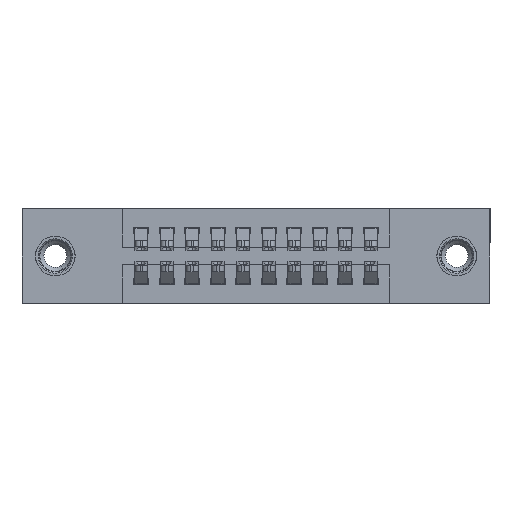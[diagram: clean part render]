
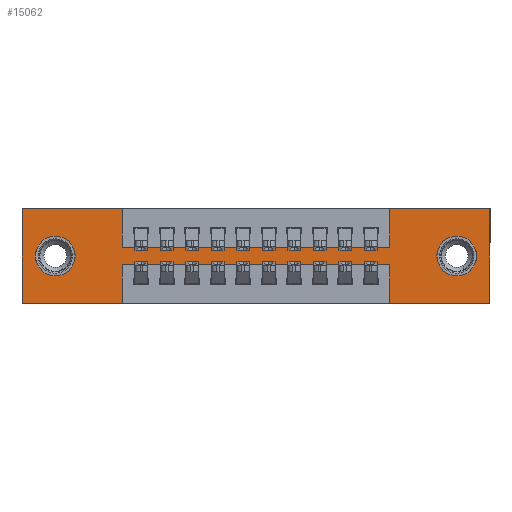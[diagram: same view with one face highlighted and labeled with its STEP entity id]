
A CAD part, front view. The second image highlights one B-rep face of the part: STEP entity #15062.
In plain terms, the highlighted planar face has unit normal (0, -1, 0).
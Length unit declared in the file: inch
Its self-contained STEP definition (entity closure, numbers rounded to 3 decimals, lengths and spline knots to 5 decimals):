
#243 = CARTESIAN_POINT ( 'NONE',  ( 0., 0., -0.37 ) ) ;
#257 = ORIENTED_EDGE ( 'NONE', *, *, #2554, .F. ) ;
#276 = ORIENTED_EDGE ( 'NONE', *, *, #4396, .F. ) ;
#324 = EDGE_LOOP ( 'NONE', ( #9780, #2620 ) ) ;
#594 = ORIENTED_EDGE ( 'NONE', *, *, #1978, .T. ) ;
#602 = LINE ( 'NONE', #3804, #6546 ) ;
#850 = FACE_OUTER_BOUND ( 'NONE', #3905, .T. ) ;
#868 = DIRECTION ( 'NONE',  ( 0., 0., -1. ) ) ;
#1363 = VERTEX_POINT ( 'NONE', #13252 ) ;
#1563 = ORIENTED_EDGE ( 'NONE', *, *, #10762, .T. ) ;
#1619 = VERTEX_POINT ( 'NONE', #2670 ) ;
#1635 = LINE ( 'NONE', #7882, #5701 ) ;
#1978 = EDGE_CURVE ( 'NONE', #2266, #1363, #8524, .T. ) ;
#2017 = LINE ( 'NONE', #12880, #12303 ) ;
#2227 = ORIENTED_EDGE ( 'NONE', *, *, #12169, .F. ) ;
#2266 = VERTEX_POINT ( 'NONE', #5858 ) ;
#2292 = CARTESIAN_POINT ( 'NONE',  ( 0.13, 0., -0.185 ) ) ;
#2314 = ORIENTED_EDGE ( 'NONE', *, *, #14480, .F. ) ;
#2331 = DIRECTION ( 'NONE',  ( 0., -1., 0. ) ) ;
#2334 = ORIENTED_EDGE ( 'NONE', *, *, #8775, .F. ) ;
#2413 = ORIENTED_EDGE ( 'NONE', *, *, #9671, .F. ) ;
#2554 = EDGE_CURVE ( 'NONE', #14967, #6202, #14658, .T. ) ;
#2620 = ORIENTED_EDGE ( 'NONE', *, *, #14324, .T. ) ;
#2665 = CARTESIAN_POINT ( 'NONE',  ( 0., 0., -0.37 ) ) ;
#2670 = CARTESIAN_POINT ( 'NONE',  ( 0.3925, 0., 0. ) ) ;
#2757 = AXIS2_PLACEMENT_3D ( 'NONE', #3664, #2331, #11707 ) ;
#2993 = ORIENTED_EDGE ( 'NONE', *, *, #8723, .F. ) ;
#3036 = LINE ( 'NONE', #13276, #5786 ) ;
#3038 = VERTEX_POINT ( 'NONE', #12413 ) ;
#3048 = CARTESIAN_POINT ( 'NONE',  ( 1.835, 0., -0.37 ) ) ;
#3061 = ORIENTED_EDGE ( 'NONE', *, *, #12995, .F. ) ;
#3322 = ORIENTED_EDGE ( 'NONE', *, *, #7286, .F. ) ;
#3502 = VECTOR ( 'NONE', #8804, 39.37008 ) ;
#3636 = AXIS2_PLACEMENT_3D ( 'NONE', #4049, #13335, #5400 ) ;
#3664 = CARTESIAN_POINT ( 'NONE',  ( 0., 0., -0.37 ) ) ;
#3687 = DIRECTION ( 'NONE',  ( 0., 0., 1. ) ) ;
#3735 = CIRCLE ( 'NONE', #12747, 0.078 ) ;
#3745 = DIRECTION ( 'NONE',  ( 0., 0., -1. ) ) ;
#3755 = AXIS2_PLACEMENT_3D ( 'NONE', #2292, #11669, #3687 ) ;
#3804 = CARTESIAN_POINT ( 'NONE',  ( 1.835, 0., 0. ) ) ;
#3808 = EDGE_CURVE ( 'NONE', #1619, #15254, #14004, .T. ) ;
#3858 = EDGE_CURVE ( 'NONE', #5129, #4149, #602, .T. ) ;
#3905 = EDGE_LOOP ( 'NONE', ( #2993, #3061, #3322, #2227, #4320, #5191, #2314, #2334, #4536, #2413, #257, #276 ) ) ;
#3941 = EDGE_LOOP ( 'NONE', ( #594, #1563 ) ) ;
#4049 = CARTESIAN_POINT ( 'NONE',  ( 0.13, 0., -0.185 ) ) ;
#4149 = VERTEX_POINT ( 'NONE', #3048 ) ;
#4315 = DIRECTION ( 'NONE',  ( -1., 0., 0. ) ) ;
#4320 = ORIENTED_EDGE ( 'NONE', *, *, #3858, .F. ) ;
#4396 = EDGE_CURVE ( 'NONE', #3038, #14967, #16436, .T. ) ;
#4428 = AXIS2_PLACEMENT_3D ( 'NONE', #5921, #6416, #868 ) ;
#4519 = CARTESIAN_POINT ( 'NONE',  ( 0.13, 0., -0.107 ) ) ;
#4536 = ORIENTED_EDGE ( 'NONE', *, *, #3808, .F. ) ;
#4612 = VERTEX_POINT ( 'NONE', #5814 ) ;
#4999 = VERTEX_POINT ( 'NONE', #14579 ) ;
#5129 = VERTEX_POINT ( 'NONE', #9556 ) ;
#5172 = DIRECTION ( 'NONE',  ( 0., 0., -1. ) ) ;
#5191 = ORIENTED_EDGE ( 'NONE', *, *, #14303, .F. ) ;
#5400 = DIRECTION ( 'NONE',  ( 0., 0., 1. ) ) ;
#5701 = VECTOR ( 'NONE', #17027, 39.37008 ) ;
#5786 = VECTOR ( 'NONE', #14714, 39.37008 ) ;
#5814 = CARTESIAN_POINT ( 'NONE',  ( 1.4425, 0., -0.15 ) ) ;
#5858 = CARTESIAN_POINT ( 'NONE',  ( 1.705, 0., -0.107 ) ) ;
#5921 = CARTESIAN_POINT ( 'NONE',  ( 1.705, 0., -0.185 ) ) ;
#6202 = VERTEX_POINT ( 'NONE', #9156 ) ;
#6337 = CARTESIAN_POINT ( 'NONE',  ( 0., 0., 0. ) ) ;
#6394 = DIRECTION ( 'NONE',  ( 0., 0., -1. ) ) ;
#6402 = CIRCLE ( 'NONE', #3636, 0.078 ) ;
#6416 = DIRECTION ( 'NONE',  ( 0., 1., 0. ) ) ;
#6546 = VECTOR ( 'NONE', #5172, 39.37008 ) ;
#6795 = CARTESIAN_POINT ( 'NONE',  ( 0.3925, 0., -0.15 ) ) ;
#7286 = EDGE_CURVE ( 'NONE', #10394, #16884, #15423, .T. ) ;
#7511 = CARTESIAN_POINT ( 'NONE',  ( 1.705, 0., -0.185 ) ) ;
#7737 = PLANE ( 'NONE',  #2757 ) ;
#7882 = CARTESIAN_POINT ( 'NONE',  ( 0.3925, 0., -0.15 ) ) ;
#7884 = LINE ( 'NONE', #6337, #14871 ) ;
#8087 = FACE_BOUND ( 'NONE', #324, .T. ) ;
#8226 = CARTESIAN_POINT ( 'NONE',  ( 1.4425, 0., -0.22 ) ) ;
#8509 = VECTOR ( 'NONE', #16335, 39.37008 ) ;
#8524 = CIRCLE ( 'NONE', #4428, 0.078 ) ;
#8605 = VERTEX_POINT ( 'NONE', #8769 ) ;
#8723 = EDGE_CURVE ( 'NONE', #11041, #3038, #9687, .T. ) ;
#8769 = CARTESIAN_POINT ( 'NONE',  ( 0.13, 0., -0.263 ) ) ;
#8775 = EDGE_CURVE ( 'NONE', #15254, #4612, #1635, .T. ) ;
#8804 = DIRECTION ( 'NONE',  ( -1., 0., 0. ) ) ;
#8850 = DIRECTION ( 'NONE',  ( 0., 0., -1. ) ) ;
#9045 = CARTESIAN_POINT ( 'NONE',  ( 1.4425, 0., -0.37 ) ) ;
#9156 = CARTESIAN_POINT ( 'NONE',  ( 0., 0., 0. ) ) ;
#9466 = DIRECTION ( 'NONE',  ( 0., 0., 1. ) ) ;
#9556 = CARTESIAN_POINT ( 'NONE',  ( 1.835, 0., 0. ) ) ;
#9671 = EDGE_CURVE ( 'NONE', #6202, #1619, #2017, .T. ) ;
#9687 = LINE ( 'NONE', #15601, #13136 ) ;
#9780 = ORIENTED_EDGE ( 'NONE', *, *, #12649, .T. ) ;
#9996 = LINE ( 'NONE', #243, #13881 ) ;
#10325 = VECTOR ( 'NONE', #12008, 39.37008 ) ;
#10394 = VERTEX_POINT ( 'NONE', #9045 ) ;
#10762 = EDGE_CURVE ( 'NONE', #1363, #2266, #3735, .T. ) ;
#11041 = VERTEX_POINT ( 'NONE', #13304 ) ;
#11388 = CIRCLE ( 'NONE', #3755, 0.078 ) ;
#11669 = DIRECTION ( 'NONE',  ( 0., 1., 0. ) ) ;
#11707 = DIRECTION ( 'NONE',  ( 0., 0., -1. ) ) ;
#11735 = CARTESIAN_POINT ( 'NONE',  ( 0.3925, 0., 0. ) ) ;
#11957 = VECTOR ( 'NONE', #9466, 39.37008 ) ;
#12008 = DIRECTION ( 'NONE',  ( -1., 0., 0. ) ) ;
#12169 = EDGE_CURVE ( 'NONE', #4149, #10394, #9996, .T. ) ;
#12303 = VECTOR ( 'NONE', #12937, 39.37008 ) ;
#12413 = CARTESIAN_POINT ( 'NONE',  ( 0.3925, 0., -0.37 ) ) ;
#12649 = EDGE_CURVE ( 'NONE', #12871, #8605, #6402, .T. ) ;
#12747 = AXIS2_PLACEMENT_3D ( 'NONE', #7511, #16661, #8850 ) ;
#12795 = CARTESIAN_POINT ( 'NONE',  ( 0., 0., -0.37 ) ) ;
#12871 = VERTEX_POINT ( 'NONE', #4519 ) ;
#12880 = CARTESIAN_POINT ( 'NONE',  ( 0., 0., 0. ) ) ;
#12937 = DIRECTION ( 'NONE',  ( 1., 0., 0. ) ) ;
#12995 = EDGE_CURVE ( 'NONE', #16884, #11041, #13699, .T. ) ;
#13136 = VECTOR ( 'NONE', #6394, 39.37008 ) ;
#13252 = CARTESIAN_POINT ( 'NONE',  ( 1.705, 0., -0.263 ) ) ;
#13276 = CARTESIAN_POINT ( 'NONE',  ( 1.4425, 0., 0. ) ) ;
#13304 = CARTESIAN_POINT ( 'NONE',  ( 0.3925, 0., -0.22 ) ) ;
#13335 = DIRECTION ( 'NONE',  ( 0., 1., 0. ) ) ;
#13699 = LINE ( 'NONE', #15363, #3502 ) ;
#13881 = VECTOR ( 'NONE', #4315, 39.37008 ) ;
#14004 = LINE ( 'NONE', #11735, #14417 ) ;
#14303 = EDGE_CURVE ( 'NONE', #4999, #5129, #7884, .T. ) ;
#14324 = EDGE_CURVE ( 'NONE', #8605, #12871, #11388, .T. ) ;
#14417 = VECTOR ( 'NONE', #3745, 39.37008 ) ;
#14480 = EDGE_CURVE ( 'NONE', #4612, #4999, #3036, .T. ) ;
#14579 = CARTESIAN_POINT ( 'NONE',  ( 1.4425, 0., 0. ) ) ;
#14650 = FACE_BOUND ( 'NONE', #3941, .T. ) ;
#14658 = LINE ( 'NONE', #16521, #8509 ) ;
#14661 = CARTESIAN_POINT ( 'NONE',  ( 1.4425, 0., -0.37 ) ) ;
#14714 = DIRECTION ( 'NONE',  ( 0., 0., 1. ) ) ;
#14871 = VECTOR ( 'NONE', #15542, 39.37008 ) ;
#14967 = VERTEX_POINT ( 'NONE', #12795 ) ;
#15062 = ADVANCED_FACE ( 'NONE', ( #14650, #8087, #850 ), #7737, .T. ) ;
#15254 = VERTEX_POINT ( 'NONE', #6795 ) ;
#15363 = CARTESIAN_POINT ( 'NONE',  ( 0.3925, 0., -0.22 ) ) ;
#15423 = LINE ( 'NONE', #14661, #11957 ) ;
#15542 = DIRECTION ( 'NONE',  ( 1., 0., 0. ) ) ;
#15601 = CARTESIAN_POINT ( 'NONE',  ( 0.3925, 0., -0.37 ) ) ;
#16335 = DIRECTION ( 'NONE',  ( 0., 0., 1. ) ) ;
#16436 = LINE ( 'NONE', #2665, #10325 ) ;
#16521 = CARTESIAN_POINT ( 'NONE',  ( 0., 0., 0. ) ) ;
#16661 = DIRECTION ( 'NONE',  ( 0., 1., 0. ) ) ;
#16884 = VERTEX_POINT ( 'NONE', #8226 ) ;
#17027 = DIRECTION ( 'NONE',  ( 1., 0., 0. ) ) ;
